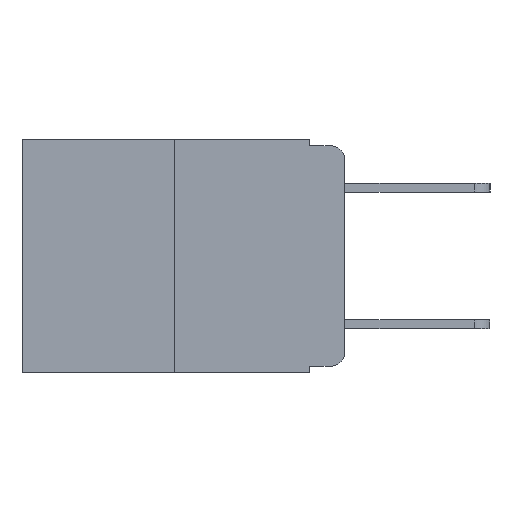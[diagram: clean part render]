
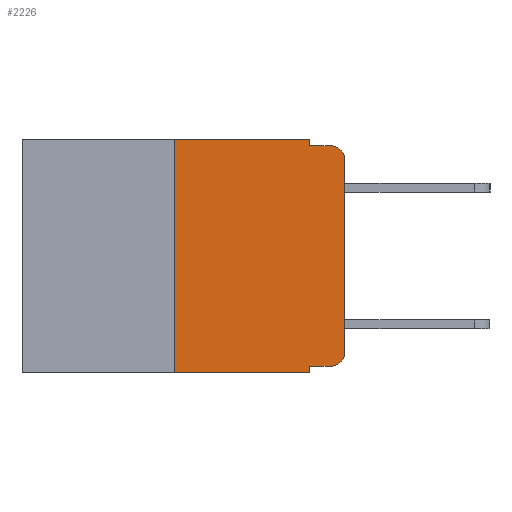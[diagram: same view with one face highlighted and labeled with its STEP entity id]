
A CAD part, left-side view. The second image highlights one B-rep face of the part: STEP entity #2226.
In plain terms, the highlighted planar face has unit normal (-1, 0, 0).
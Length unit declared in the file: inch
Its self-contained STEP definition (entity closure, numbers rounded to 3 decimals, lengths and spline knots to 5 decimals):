
#163 = VERTEX_POINT ( 'NONE', #16655 ) ;
#185 = EDGE_LOOP ( 'NONE', ( #16996, #17390, #10970, #15140, #532, #4658, #16003, #7330, #1742, #14301 ) ) ;
#323 = EDGE_CURVE ( 'NONE', #12341, #2774, #12497, .T. ) ;
#397 = VECTOR ( 'NONE', #5898, 39.37008 ) ;
#532 = ORIENTED_EDGE ( 'NONE', *, *, #6803, .F. ) ;
#563 = VECTOR ( 'NONE', #9812, 39.37008 ) ;
#1166 = DIRECTION ( 'NONE',  ( -1., 0., 0. ) ) ;
#1468 = CARTESIAN_POINT ( 'NONE',  ( 0., 0.02, -0.313 ) ) ;
#1742 = ORIENTED_EDGE ( 'NONE', *, *, #3841, .T. ) ;
#2226 = ADVANCED_FACE ( 'NONE', ( #8169 ), #7987, .F. ) ;
#2385 = CARTESIAN_POINT ( 'NONE',  ( 0., 0.051, 0. ) ) ;
#2774 = VERTEX_POINT ( 'NONE', #15468 ) ;
#2818 = EDGE_CURVE ( 'NONE', #12999, #3197, #7198, .T. ) ;
#2971 = EDGE_CURVE ( 'NONE', #13498, #4173, #12202, .T. ) ;
#3122 = VECTOR ( 'NONE', #15228, 39.37008 ) ;
#3197 = VERTEX_POINT ( 'NONE', #6132 ) ;
#3659 = LINE ( 'NONE', #16307, #7076 ) ;
#3841 = EDGE_CURVE ( 'NONE', #14622, #12999, #11309, .T. ) ;
#4173 = VERTEX_POINT ( 'NONE', #12756 ) ;
#4658 = ORIENTED_EDGE ( 'NONE', *, *, #9717, .F. ) ;
#4688 = LINE ( 'NONE', #2385, #563 ) ;
#4713 = DIRECTION ( 'NONE',  ( 0., 0., 1. ) ) ;
#4864 = DIRECTION ( 'NONE',  ( -1., 0., 0. ) ) ;
#5066 = CARTESIAN_POINT ( 'NONE',  ( 0., 0.051, -0.333 ) ) ;
#5179 = CARTESIAN_POINT ( 'NONE',  ( 0., 0.051, 0. ) ) ;
#5407 = AXIS2_PLACEMENT_3D ( 'NONE', #9434, #4864, #12421 ) ;
#5458 = EDGE_CURVE ( 'NONE', #3197, #12341, #3659, .T. ) ;
#5499 = DIRECTION ( 'NONE',  ( 0., -1., 0. ) ) ;
#5550 = CARTESIAN_POINT ( 'NONE',  ( 0., 0.051, -0.01 ) ) ;
#5898 = DIRECTION ( 'NONE',  ( 0., -1., 0. ) ) ;
#6132 = CARTESIAN_POINT ( 'NONE',  ( 0., 0., -0.313 ) ) ;
#6244 = DIRECTION ( 'NONE',  ( 0., 0., -1. ) ) ;
#6698 = CARTESIAN_POINT ( 'NONE',  ( 0., 0.473, 0. ) ) ;
#6777 = EDGE_CURVE ( 'NONE', #14622, #4173, #11799, .T. ) ;
#6803 = EDGE_CURVE ( 'NONE', #163, #11820, #15069, .T. ) ;
#6994 = VECTOR ( 'NONE', #5499, 39.37008 ) ;
#7076 = VECTOR ( 'NONE', #8417, 39.37008 ) ;
#7198 = CIRCLE ( 'NONE', #13161, 0.02 ) ;
#7234 = DIRECTION ( 'NONE',  ( 0., -1., 0. ) ) ;
#7272 = CARTESIAN_POINT ( 'NONE',  ( 0., 0.25, -0.343 ) ) ;
#7330 = ORIENTED_EDGE ( 'NONE', *, *, #6777, .F. ) ;
#7418 = CARTESIAN_POINT ( 'NONE',  ( 0., 0.02, -0.333 ) ) ;
#7457 = VECTOR ( 'NONE', #9556, 39.37008 ) ;
#7987 = PLANE ( 'NONE',  #15686 ) ;
#8169 = FACE_OUTER_BOUND ( 'NONE', #185, .T. ) ;
#8358 = CARTESIAN_POINT ( 'NONE',  ( 0., 0.473, -0.343 ) ) ;
#8417 = DIRECTION ( 'NONE',  ( 0., 0., 1. ) ) ;
#8872 = VECTOR ( 'NONE', #7234, 39.37008 ) ;
#9172 = DIRECTION ( 'NONE',  ( 0., 0., -1. ) ) ;
#9434 = CARTESIAN_POINT ( 'NONE',  ( 0., 0.02, -0.03 ) ) ;
#9556 = DIRECTION ( 'NONE',  ( 0., 0., -1. ) ) ;
#9639 = DIRECTION ( 'NONE',  ( 1., 0., 0. ) ) ;
#9717 = EDGE_CURVE ( 'NONE', #13498, #163, #13037, .T. ) ;
#9812 = DIRECTION ( 'NONE',  ( 0., 0., -1. ) ) ;
#10401 = CARTESIAN_POINT ( 'NONE',  ( 0., 0., -0.03 ) ) ;
#10473 = CARTESIAN_POINT ( 'NONE',  ( 0., 0.25, 0. ) ) ;
#10661 = EDGE_CURVE ( 'NONE', #11820, #13383, #4688, .T. ) ;
#10970 = ORIENTED_EDGE ( 'NONE', *, *, #14444, .F. ) ;
#11309 = LINE ( 'NONE', #11667, #6994 ) ;
#11667 = CARTESIAN_POINT ( 'NONE',  ( 0., 0.051, -0.333 ) ) ;
#11799 = LINE ( 'NONE', #5179, #7457 ) ;
#11820 = VERTEX_POINT ( 'NONE', #15840 ) ;
#12202 = LINE ( 'NONE', #8358, #397 ) ;
#12341 = VERTEX_POINT ( 'NONE', #10401 ) ;
#12421 = DIRECTION ( 'NONE',  ( 0., 0., -1. ) ) ;
#12472 = CARTESIAN_POINT ( 'NONE',  ( 0., 0.473, 0. ) ) ;
#12497 = CIRCLE ( 'NONE', #5407, 0.02 ) ;
#12582 = VECTOR ( 'NONE', #4713, 39.37008 ) ;
#12692 = LINE ( 'NONE', #13011, #8872 ) ;
#12756 = CARTESIAN_POINT ( 'NONE',  ( 0., 0.051, -0.343 ) ) ;
#12999 = VERTEX_POINT ( 'NONE', #7418 ) ;
#13011 = CARTESIAN_POINT ( 'NONE',  ( 0., 0.051, -0.01 ) ) ;
#13037 = LINE ( 'NONE', #10473, #12582 ) ;
#13161 = AXIS2_PLACEMENT_3D ( 'NONE', #1468, #1166, #6244 ) ;
#13383 = VERTEX_POINT ( 'NONE', #5550 ) ;
#13498 = VERTEX_POINT ( 'NONE', #7272 ) ;
#14301 = ORIENTED_EDGE ( 'NONE', *, *, #2818, .T. ) ;
#14444 = EDGE_CURVE ( 'NONE', #13383, #2774, #12692, .T. ) ;
#14622 = VERTEX_POINT ( 'NONE', #5066 ) ;
#15069 = LINE ( 'NONE', #6698, #3122 ) ;
#15140 = ORIENTED_EDGE ( 'NONE', *, *, #10661, .F. ) ;
#15228 = DIRECTION ( 'NONE',  ( 0., -1., 0. ) ) ;
#15468 = CARTESIAN_POINT ( 'NONE',  ( 0., 0.02, -0.01 ) ) ;
#15686 = AXIS2_PLACEMENT_3D ( 'NONE', #12472, #9639, #9172 ) ;
#15840 = CARTESIAN_POINT ( 'NONE',  ( 0., 0.051, 0. ) ) ;
#16003 = ORIENTED_EDGE ( 'NONE', *, *, #2971, .T. ) ;
#16307 = CARTESIAN_POINT ( 'NONE',  ( 0., 0., 0. ) ) ;
#16655 = CARTESIAN_POINT ( 'NONE',  ( 0., 0.25, 0. ) ) ;
#16996 = ORIENTED_EDGE ( 'NONE', *, *, #5458, .T. ) ;
#17390 = ORIENTED_EDGE ( 'NONE', *, *, #323, .T. ) ;
